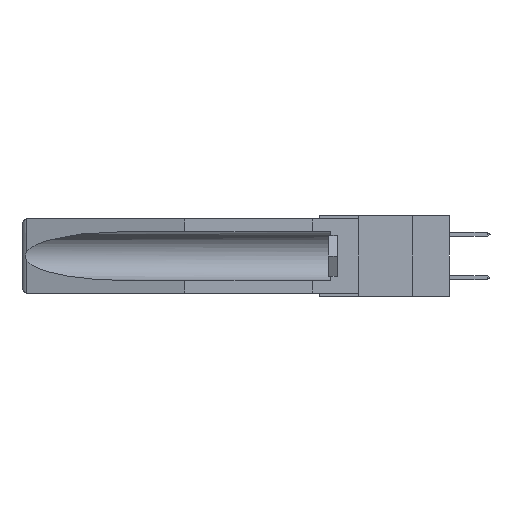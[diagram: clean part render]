
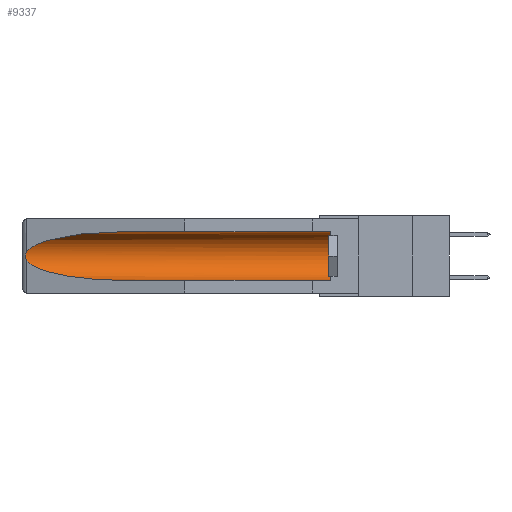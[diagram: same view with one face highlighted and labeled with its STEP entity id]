
A CAD part, left-side view. The second image highlights one B-rep face of the part: STEP entity #9337.
In plain terms, the highlighted cylindrical face has radius 2.857 mm (diameter 5.715 mm), a partial arc.
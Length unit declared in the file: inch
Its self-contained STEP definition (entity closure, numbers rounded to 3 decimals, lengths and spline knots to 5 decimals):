
#181 = CARTESIAN_POINT ( 'NONE',  ( 0.155, 1.07973, -0.284 ) ) ;
#362 = CARTESIAN_POINT ( 'NONE',  ( 0.25451, 1.48313, -0.24835 ) ) ;
#477 = ORIENTED_EDGE ( 'NONE', *, *, #4957, .F. ) ;
#649 = EDGE_LOOP ( 'NONE', ( #10737, #6223, #15709, #477, #15829, #19782 ) ) ;
#1294 = CARTESIAN_POINT ( 'NONE',  ( 0.26537, 1.52718, -0.19328 ) ) ;
#1543 = CARTESIAN_POINT ( 'NONE',  ( 0.155, 1.07973, -0.059 ) ) ;
#1572 = CARTESIAN_POINT ( 'NONE',  ( 0.26537, 1.52718, -0.14972 ) ) ;
#1717 = CARTESIAN_POINT ( 'NONE',  ( 0.26537, 1.52718, -0.14972 ) ) ;
#1803 = VERTEX_POINT ( 'NONE', #5092 ) ;
#2433 = CARTESIAN_POINT ( 'NONE',  ( 0.155, -0.30754, -0.284 ) ) ;
#2746 = VECTOR ( 'NONE', #12979, 39.37008 ) ;
#2899 = CARTESIAN_POINT ( 'NONE',  ( 0.26654, 1.53092, -0.15636 ) ) ;
#3049 = CARTESIAN_POINT ( 'NONE',  ( 0.2675, 1.53308, -0.17534 ) ) ;
#3604 = CYLINDRICAL_SURFACE ( 'NONE', #15667, 0.1125 ) ;
#4555 = LINE ( 'NONE', #2433, #17495 ) ;
#4957 = EDGE_CURVE ( 'NONE', #1803, #14486, #4555, .T. ) ;
#5092 = CARTESIAN_POINT ( 'NONE',  ( 0.155, 0.126, -0.284 ) ) ;
#5477 = DIRECTION ( 'NONE',  ( 0., 0., 1. ) ) ;
#6080 = CARTESIAN_POINT ( 'NONE',  ( 0.155, -0.30754, -0.059 ) ) ;
#6223 = ORIENTED_EDGE ( 'NONE', *, *, #19274, .T. ) ;
#6316 = VERTEX_POINT ( 'NONE', #19726 ) ;
#6377 = CARTESIAN_POINT ( 'NONE',  ( 0.2673, 1.53269, -0.17917 ) ) ;
#6517 = CARTESIAN_POINT ( 'NONE',  ( 0.2673, 1.5327, -0.16383 ) ) ;
#7480 = VERTEX_POINT ( 'NONE', #15996 ) ;
#7715 = DIRECTION ( 'NONE',  ( 0., 0., 1. ) ) ;
#9337 = ADVANCED_FACE ( 'NONE', ( #13038 ), #3604, .F. ) ;
#9998 = CARTESIAN_POINT ( 'NONE',  ( 0.21114, 1.30732, -0.059 ) ) ;
#10026 = EDGE_CURVE ( 'NONE', #7480, #11705, #16503, .T. ) ;
#10159 = CARTESIAN_POINT ( 'NONE',  ( 0.155, 1.07973, -0.059 ) ) ;
#10737 = ORIENTED_EDGE ( 'NONE', *, *, #17222, .T. ) ;
#11705 = VERTEX_POINT ( 'NONE', #1543 ) ;
#12170 = EDGE_CURVE ( 'NONE', #1803, #7480, #13953, .T. ) ;
#12439 = CARTESIAN_POINT ( 'NONE',  ( 0.155, 1.07973, -0.284 ) ) ;
#12979 = DIRECTION ( 'NONE',  ( 0., 1., 0. ) ) ;
#13038 = FACE_OUTER_BOUND ( 'NONE', #649, .T. ) ;
#13179 = EDGE_CURVE ( 'NONE', #6316, #14486, #15206, .T. ) ;
#13206 = CARTESIAN_POINT ( 'NONE',  ( 0.26597, 1.52961, -0.15275 ) ) ;
#13282 = CARTESIAN_POINT ( 'NONE',  ( 0.2675, 1.53308, -0.16763 ) ) ;
#13953 = CIRCLE ( 'NONE', #22299, 0.1125 ) ;
#14482 =( BOUNDED_CURVE ( )  B_SPLINE_CURVE ( 3, ( #10159, #9998, #15370, #1717 ),
 .UNSPECIFIED., .F., .T. ) 
 B_SPLINE_CURVE_WITH_KNOTS ( ( 4, 4 ),
 ( 4.71239, 6.08839 ),
 .UNSPECIFIED. ) 
 CURVE ( )  GEOMETRIC_REPRESENTATION_ITEM ( )  RATIONAL_B_SPLINE_CURVE ( ( 1., 0.848, 0.848, 1. ) ) 
 REPRESENTATION_ITEM ( '' )  );
#14486 = VERTEX_POINT ( 'NONE', #181 ) ;
#14503 = DIRECTION ( 'NONE',  ( 0., 1., 0. ) ) ;
#14787 = CARTESIAN_POINT ( 'NONE',  ( 0.26655, 1.53094, -0.18657 ) ) ;
#15202 = CARTESIAN_POINT ( 'NONE',  ( 0.155, -0.30754, -0.1715 ) ) ;
#15206 =( BOUNDED_CURVE ( )  B_SPLINE_CURVE ( 3, ( #17784, #362, #21139, #12439 ),
 .UNSPECIFIED., .F., .F. ) 
 B_SPLINE_CURVE_WITH_KNOTS ( ( 4, 4 ),
 ( 0.1948, 1.5708 ),
 .UNSPECIFIED. ) 
 CURVE ( )  GEOMETRIC_REPRESENTATION_ITEM ( )  RATIONAL_B_SPLINE_CURVE ( ( 1., 0.848, 0.848, 1. ) ) 
 REPRESENTATION_ITEM ( '' )  );
#15370 = CARTESIAN_POINT ( 'NONE',  ( 0.25451, 1.48313, -0.09465 ) ) ;
#15667 = AXIS2_PLACEMENT_3D ( 'NONE', #15202, #18675, #5477 ) ;
#15709 = ORIENTED_EDGE ( 'NONE', *, *, #13179, .T. ) ;
#15829 = ORIENTED_EDGE ( 'NONE', *, *, #12170, .T. ) ;
#15996 = CARTESIAN_POINT ( 'NONE',  ( 0.155, 0.126, -0.059 ) ) ;
#16434 = CARTESIAN_POINT ( 'NONE',  ( 0.155, 0.126, -0.1715 ) ) ;
#16503 = LINE ( 'NONE', #6080, #2746 ) ;
#16536 = CARTESIAN_POINT ( 'NONE',  ( 0.26597, 1.5296, -0.19026 ) ) ;
#17222 = EDGE_CURVE ( 'NONE', #11705, #20147, #14482, .T. ) ;
#17495 = VECTOR ( 'NONE', #14503, 39.37008 ) ;
#17521 = B_SPLINE_CURVE_WITH_KNOTS ( 'NONE', 3,
 ( #20106, #13206, #2899, #6517, #13282, #3049, #6377, #14787, #16536, #1294 ),
 .UNSPECIFIED., .F., .F.,
 ( 4, 2, 2, 2, 4 ),
 ( 0., 0.00029, 0.00058, 0.00087, 0.00117 ),
 .UNSPECIFIED. ) ;
#17784 = CARTESIAN_POINT ( 'NONE',  ( 0.26537, 1.52718, -0.19328 ) ) ;
#18675 = DIRECTION ( 'NONE',  ( 0., 1., 0. ) ) ;
#19274 = EDGE_CURVE ( 'NONE', #20147, #6316, #17521, .T. ) ;
#19726 = CARTESIAN_POINT ( 'NONE',  ( 0.26537, 1.52718, -0.19328 ) ) ;
#19782 = ORIENTED_EDGE ( 'NONE', *, *, #10026, .T. ) ;
#20106 = CARTESIAN_POINT ( 'NONE',  ( 0.26537, 1.52718, -0.14972 ) ) ;
#20147 = VERTEX_POINT ( 'NONE', #1572 ) ;
#21139 = CARTESIAN_POINT ( 'NONE',  ( 0.21114, 1.30732, -0.284 ) ) ;
#21440 = DIRECTION ( 'NONE',  ( 0., -1., 0. ) ) ;
#22299 = AXIS2_PLACEMENT_3D ( 'NONE', #16434, #21440, #7715 ) ;
